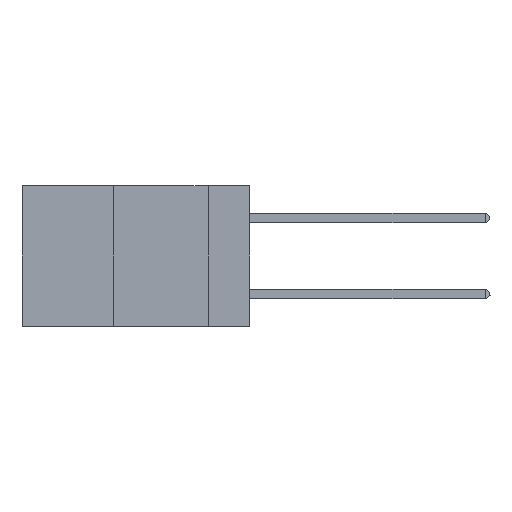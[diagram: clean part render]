
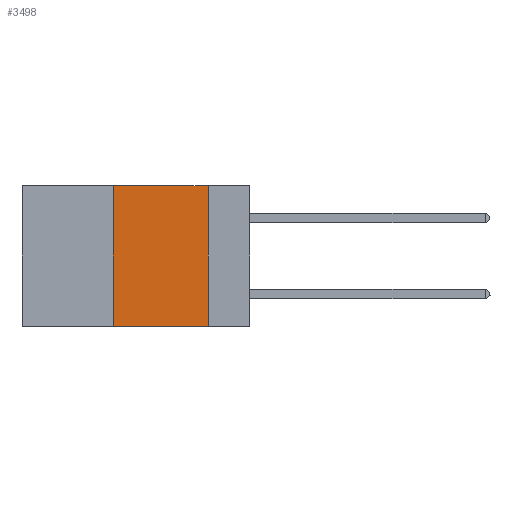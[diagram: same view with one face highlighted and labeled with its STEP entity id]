
A CAD part, left-side view. The second image highlights one B-rep face of the part: STEP entity #3498.
In plain terms, the highlighted planar face has unit normal (-1, 0, 0).
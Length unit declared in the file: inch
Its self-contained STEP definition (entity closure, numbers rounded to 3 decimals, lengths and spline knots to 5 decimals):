
#339 = DIRECTION ( 'NONE',  ( 1., 0., 0. ) ) ;
#1224 = VECTOR ( 'NONE', #8683, 39.37008 ) ;
#1642 = LINE ( 'NONE', #3025, #3525 ) ;
#2659 = LINE ( 'NONE', #3383, #9526 ) ;
#3025 = CARTESIAN_POINT ( 'NONE',  ( 0., 0.6, 0. ) ) ;
#3383 = CARTESIAN_POINT ( 'NONE',  ( 0., 0.6, -0.37 ) ) ;
#3498 = ADVANCED_FACE ( 'NONE', ( #17781 ), #15121, .F. ) ;
#3525 = VECTOR ( 'NONE', #9089, 39.37008 ) ;
#3607 = CARTESIAN_POINT ( 'NONE',  ( 0., 0.11, -0.37 ) ) ;
#5227 = VERTEX_POINT ( 'NONE', #11154 ) ;
#6187 = CARTESIAN_POINT ( 'NONE',  ( 0., 0.6, 0. ) ) ;
#7376 = VERTEX_POINT ( 'NONE', #14369 ) ;
#7750 = DIRECTION ( 'NONE',  ( 0., -1., 0. ) ) ;
#7784 = EDGE_CURVE ( 'NONE', #5227, #8086, #2659, .T. ) ;
#8037 = DIRECTION ( 'NONE',  ( 0., 0., -1. ) ) ;
#8086 = VERTEX_POINT ( 'NONE', #3607 ) ;
#8462 = CARTESIAN_POINT ( 'NONE',  ( 0., 0.11, 0. ) ) ;
#8683 = DIRECTION ( 'NONE',  ( 0., 0., 1. ) ) ;
#8706 = ORIENTED_EDGE ( 'NONE', *, *, #7784, .T. ) ;
#9089 = DIRECTION ( 'NONE',  ( 0., -1., 0. ) ) ;
#9526 = VECTOR ( 'NONE', #7750, 39.37008 ) ;
#9879 = ORIENTED_EDGE ( 'NONE', *, *, #15389, .F. ) ;
#10238 = EDGE_CURVE ( 'NONE', #7376, #16830, #1642, .T. ) ;
#11154 = CARTESIAN_POINT ( 'NONE',  ( 0., 0.36, -0.37 ) ) ;
#12457 = LINE ( 'NONE', #14541, #15712 ) ;
#13176 = AXIS2_PLACEMENT_3D ( 'NONE', #6187, #339, #8037 ) ;
#14369 = CARTESIAN_POINT ( 'NONE',  ( 0., 0.36, 0. ) ) ;
#14420 = DIRECTION ( 'NONE',  ( 0., 0., -1. ) ) ;
#14541 = CARTESIAN_POINT ( 'NONE',  ( 0., 0.11, 0. ) ) ;
#14964 = EDGE_LOOP ( 'NONE', ( #18227, #17312, #9879, #8706 ) ) ;
#15121 = PLANE ( 'NONE',  #13176 ) ;
#15389 = EDGE_CURVE ( 'NONE', #5227, #7376, #18758, .T. ) ;
#15712 = VECTOR ( 'NONE', #14420, 39.37008 ) ;
#15898 = CARTESIAN_POINT ( 'NONE',  ( 0., 0.36, 0. ) ) ;
#16076 = EDGE_CURVE ( 'NONE', #16830, #8086, #12457, .T. ) ;
#16830 = VERTEX_POINT ( 'NONE', #8462 ) ;
#17312 = ORIENTED_EDGE ( 'NONE', *, *, #10238, .F. ) ;
#17781 = FACE_OUTER_BOUND ( 'NONE', #14964, .T. ) ;
#18227 = ORIENTED_EDGE ( 'NONE', *, *, #16076, .F. ) ;
#18758 = LINE ( 'NONE', #15898, #1224 ) ;
